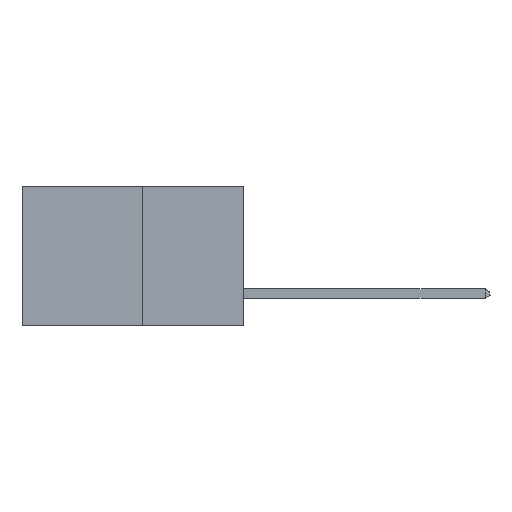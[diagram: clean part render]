
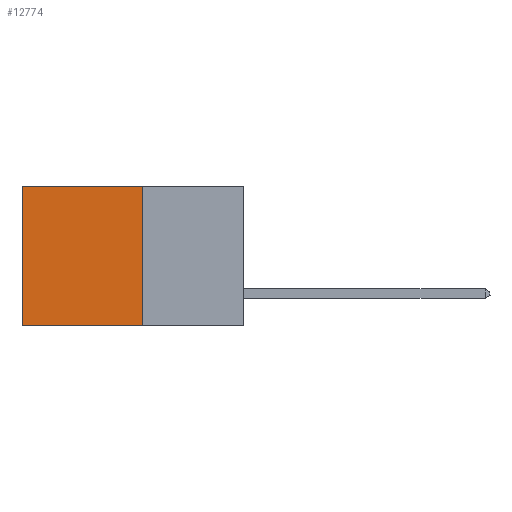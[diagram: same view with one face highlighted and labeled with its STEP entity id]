
A CAD part, left-side view. The second image highlights one B-rep face of the part: STEP entity #12774.
In plain terms, the highlighted planar face has unit normal (-1, 0, 0).
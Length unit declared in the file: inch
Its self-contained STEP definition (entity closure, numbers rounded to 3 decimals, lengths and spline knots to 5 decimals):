
#73 = EDGE_CURVE ( 'NONE', #8835, #4616, #3959, .T. ) ;
#151 = PLANE ( 'NONE',  #5637 ) ;
#781 = FACE_OUTER_BOUND ( 'NONE', #7997, .T. ) ;
#1169 = VERTEX_POINT ( 'NONE', #11610 ) ;
#1215 = CARTESIAN_POINT ( 'NONE',  ( 0.277, 0.27, -0.37 ) ) ;
#1369 = DIRECTION ( 'NONE',  ( 1., 0., 0. ) ) ;
#1785 = CARTESIAN_POINT ( 'NONE',  ( 0.277, 0.27, 0. ) ) ;
#2454 = CARTESIAN_POINT ( 'NONE',  ( 0.277, 0.59, -0.37 ) ) ;
#2797 = EDGE_CURVE ( 'NONE', #8835, #1169, #6957, .T. ) ;
#2893 = DIRECTION ( 'NONE',  ( 0., 1., 0. ) ) ;
#3439 = DIRECTION ( 'NONE',  ( 0., 0., -1. ) ) ;
#3959 = LINE ( 'NONE', #4507, #12382 ) ;
#4507 = CARTESIAN_POINT ( 'NONE',  ( 0.277, 0.27, -0.37 ) ) ;
#4616 = VERTEX_POINT ( 'NONE', #1215 ) ;
#5637 = AXIS2_PLACEMENT_3D ( 'NONE', #11417, #1369, #9349 ) ;
#6957 = LINE ( 'NONE', #1785, #7321 ) ;
#7100 = DIRECTION ( 'NONE',  ( 0., 0., -1. ) ) ;
#7321 = VECTOR ( 'NONE', #13377, 39.37008 ) ;
#7747 = EDGE_CURVE ( 'NONE', #4616, #13402, #13076, .T. ) ;
#7997 = EDGE_LOOP ( 'NONE', ( #9938, #10287, #12979, #10628 ) ) ;
#8044 = CARTESIAN_POINT ( 'NONE',  ( 0.277, 0.27, -0.37 ) ) ;
#8123 = VECTOR ( 'NONE', #3439, 39.37008 ) ;
#8835 = VERTEX_POINT ( 'NONE', #11442 ) ;
#9349 = DIRECTION ( 'NONE',  ( 0., 0., -1. ) ) ;
#9938 = ORIENTED_EDGE ( 'NONE', *, *, #13705, .T. ) ;
#10287 = ORIENTED_EDGE ( 'NONE', *, *, #7747, .F. ) ;
#10368 = VECTOR ( 'NONE', #2893, 39.37008 ) ;
#10628 = ORIENTED_EDGE ( 'NONE', *, *, #2797, .T. ) ;
#11417 = CARTESIAN_POINT ( 'NONE',  ( 0.277, 0.27, -0.37 ) ) ;
#11442 = CARTESIAN_POINT ( 'NONE',  ( 0.277, 0.27, 0. ) ) ;
#11610 = CARTESIAN_POINT ( 'NONE',  ( 0.277, 0.59, 0. ) ) ;
#12267 = CARTESIAN_POINT ( 'NONE',  ( 0.277, 0.59, -0.37 ) ) ;
#12382 = VECTOR ( 'NONE', #7100, 39.37008 ) ;
#12774 = ADVANCED_FACE ( 'NONE', ( #781 ), #151, .F. ) ;
#12979 = ORIENTED_EDGE ( 'NONE', *, *, #73, .F. ) ;
#13076 = LINE ( 'NONE', #8044, #10368 ) ;
#13377 = DIRECTION ( 'NONE',  ( 0., 1., 0. ) ) ;
#13402 = VERTEX_POINT ( 'NONE', #2454 ) ;
#13705 = EDGE_CURVE ( 'NONE', #1169, #13402, #14070, .T. ) ;
#14070 = LINE ( 'NONE', #12267, #8123 ) ;
